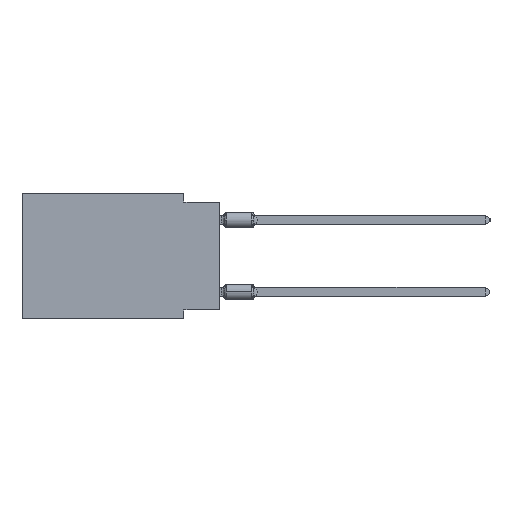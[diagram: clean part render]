
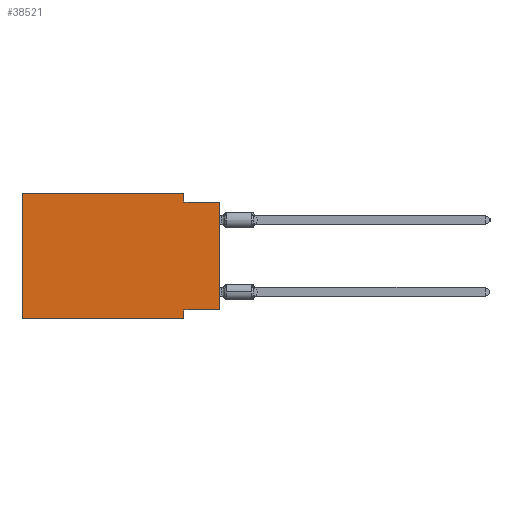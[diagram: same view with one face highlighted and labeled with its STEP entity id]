
A CAD part, left-side view. The second image highlights one B-rep face of the part: STEP entity #38521.
In plain terms, the highlighted planar face has unit normal (-1, 0, 0).
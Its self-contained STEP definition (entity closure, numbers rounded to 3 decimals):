
#75 = VERTEX_POINT ( 'NONE', #48863 ) ;
#1179 = ORIENTED_EDGE ( 'NONE', *, *, #60717, .F. ) ;
#2877 = CARTESIAN_POINT ( 'NONE',  ( 0., 13.97, -8.89 ) ) ;
#3942 = CARTESIAN_POINT ( 'NONE',  ( 0., 2.54, -0.635 ) ) ;
#5902 = EDGE_LOOP ( 'NONE', ( #54151, #7768, #1179, #48658, #22927, #14901, #29411, #6635 ) ) ;
#6635 = ORIENTED_EDGE ( 'NONE', *, *, #10721, .F. ) ;
#7768 = ORIENTED_EDGE ( 'NONE', *, *, #58263, .F. ) ;
#8441 = VECTOR ( 'NONE', #9636, 1000. ) ;
#8576 = PLANE ( 'NONE',  #38397 ) ;
#9636 = DIRECTION ( 'NONE',  ( 0., -1., 0. ) ) ;
#10088 = VERTEX_POINT ( 'NONE', #2877 ) ;
#10686 = CARTESIAN_POINT ( 'NONE',  ( 0., 13.97, 0. ) ) ;
#10721 = EDGE_CURVE ( 'NONE', #30324, #75, #14896, .T. ) ;
#12874 = CARTESIAN_POINT ( 'NONE',  ( 0., 0., -0.635 ) ) ;
#14896 = LINE ( 'NONE', #24427, #58335 ) ;
#14901 = ORIENTED_EDGE ( 'NONE', *, *, #51355, .T. ) ;
#14984 = EDGE_CURVE ( 'NONE', #10088, #41625, #20624, .T. ) ;
#15977 = LINE ( 'NONE', #50027, #51230 ) ;
#16162 = CARTESIAN_POINT ( 'NONE',  ( 0., 13.97, 0. ) ) ;
#16347 = VERTEX_POINT ( 'NONE', #29883 ) ;
#19671 = DIRECTION ( 'NONE',  ( 0., 1., 0. ) ) ;
#19876 = EDGE_CURVE ( 'NONE', #30324, #24790, #39203, .T. ) ;
#20624 = LINE ( 'NONE', #16162, #49433 ) ;
#21385 = VECTOR ( 'NONE', #52574, 1000. ) ;
#21447 = DIRECTION ( 'NONE',  ( 0., 0., -1. ) ) ;
#22924 = DIRECTION ( 'NONE',  ( 1., 0., 0. ) ) ;
#22927 = ORIENTED_EDGE ( 'NONE', *, *, #14984, .F. ) ;
#24427 = CARTESIAN_POINT ( 'NONE',  ( 0., 0., -8.255 ) ) ;
#24790 = VERTEX_POINT ( 'NONE', #41805 ) ;
#26726 = VECTOR ( 'NONE', #21447, 1000. ) ;
#29345 = CARTESIAN_POINT ( 'NONE',  ( 0., 0., 0. ) ) ;
#29411 = ORIENTED_EDGE ( 'NONE', *, *, #61262, .F. ) ;
#29883 = CARTESIAN_POINT ( 'NONE',  ( 0., 2.54, 0. ) ) ;
#29976 = DIRECTION ( 'NONE',  ( 0., 0., -1. ) ) ;
#30324 = VERTEX_POINT ( 'NONE', #42593 ) ;
#35463 = CARTESIAN_POINT ( 'NONE',  ( 0., 2.54, 0. ) ) ;
#37060 = LINE ( 'NONE', #12874, #57051 ) ;
#38005 = DIRECTION ( 'NONE',  ( 0., 0., 1. ) ) ;
#38397 = AXIS2_PLACEMENT_3D ( 'NONE', #56976, #22924, #53144 ) ;
#38521 = ADVANCED_FACE ( 'NONE', ( #42022 ), #8576, .F. ) ;
#39203 = LINE ( 'NONE', #29345, #51557 ) ;
#39244 = LINE ( 'NONE', #58347, #8441 ) ;
#41521 = DIRECTION ( 'NONE',  ( 0., -1., 0. ) ) ;
#41625 = VERTEX_POINT ( 'NONE', #10686 ) ;
#41805 = CARTESIAN_POINT ( 'NONE',  ( 0., 0., -0.635 ) ) ;
#42022 = FACE_OUTER_BOUND ( 'NONE', #5902, .T. ) ;
#42593 = CARTESIAN_POINT ( 'NONE',  ( 0., 0., -8.255 ) ) ;
#45332 = VERTEX_POINT ( 'NONE', #3942 ) ;
#47322 = CARTESIAN_POINT ( 'NONE',  ( 0., 2.54, -8.89 ) ) ;
#47795 = LINE ( 'NONE', #62430, #21385 ) ;
#48658 = ORIENTED_EDGE ( 'NONE', *, *, #57554, .F. ) ;
#48863 = CARTESIAN_POINT ( 'NONE',  ( 0., 2.54, -8.255 ) ) ;
#49433 = VECTOR ( 'NONE', #49893, 1000. ) ;
#49893 = DIRECTION ( 'NONE',  ( 0., 0., 1. ) ) ;
#50027 = CARTESIAN_POINT ( 'NONE',  ( 0., 2.54, -8.89 ) ) ;
#51230 = VECTOR ( 'NONE', #29976, 1000. ) ;
#51355 = EDGE_CURVE ( 'NONE', #10088, #53860, #39244, .T. ) ;
#51557 = VECTOR ( 'NONE', #38005, 1000. ) ;
#52574 = DIRECTION ( 'NONE',  ( 0., -1., 0. ) ) ;
#53144 = DIRECTION ( 'NONE',  ( 0., 0., -1. ) ) ;
#53860 = VERTEX_POINT ( 'NONE', #47322 ) ;
#54151 = ORIENTED_EDGE ( 'NONE', *, *, #19876, .T. ) ;
#54870 = LINE ( 'NONE', #35463, #26726 ) ;
#56976 = CARTESIAN_POINT ( 'NONE',  ( 0., 13.97, 0. ) ) ;
#57051 = VECTOR ( 'NONE', #41521, 1000. ) ;
#57554 = EDGE_CURVE ( 'NONE', #41625, #16347, #47795, .T. ) ;
#58263 = EDGE_CURVE ( 'NONE', #45332, #24790, #37060, .T. ) ;
#58335 = VECTOR ( 'NONE', #19671, 1000. ) ;
#58347 = CARTESIAN_POINT ( 'NONE',  ( 0., 13.97, -8.89 ) ) ;
#60717 = EDGE_CURVE ( 'NONE', #16347, #45332, #54870, .T. ) ;
#61262 = EDGE_CURVE ( 'NONE', #75, #53860, #15977, .T. ) ;
#62430 = CARTESIAN_POINT ( 'NONE',  ( 0., 13.97, 0. ) ) ;
